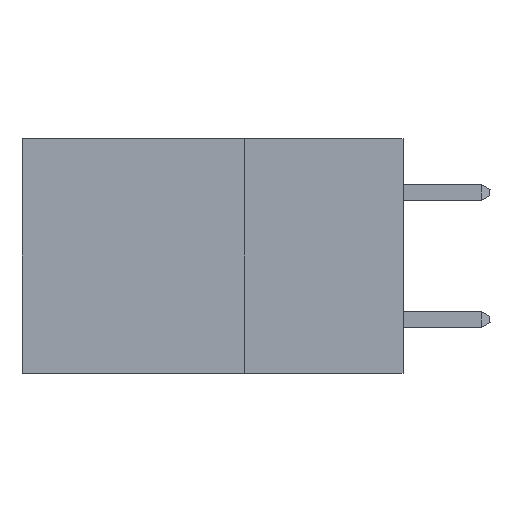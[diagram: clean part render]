
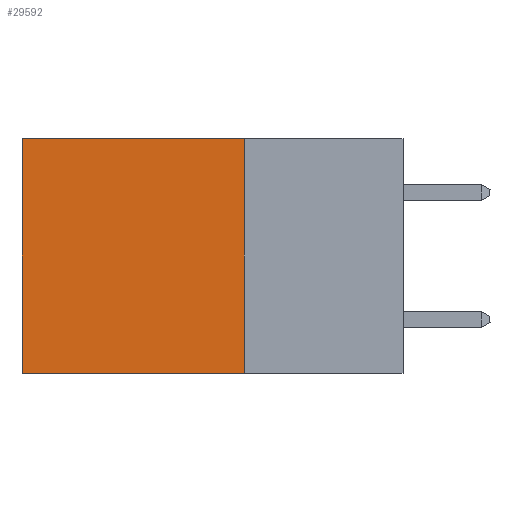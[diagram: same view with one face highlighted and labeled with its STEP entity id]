
A CAD part, left-side view. The second image highlights one B-rep face of the part: STEP entity #29592.
In plain terms, the highlighted planar face has unit normal (-1, 0, 0).
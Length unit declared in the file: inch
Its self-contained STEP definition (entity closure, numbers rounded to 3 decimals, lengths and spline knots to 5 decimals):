
#1355 = ORIENTED_EDGE ( 'NONE', *, *, #19962, .T. ) ;
#1936 = FACE_OUTER_BOUND ( 'NONE', #5092, .T. ) ;
#2747 = VECTOR ( 'NONE', #10134, 39.37008 ) ;
#3087 = DIRECTION ( 'NONE',  ( 0., 1., 0. ) ) ;
#3748 = VECTOR ( 'NONE', #14158, 39.37008 ) ;
#5092 = EDGE_LOOP ( 'NONE', ( #1355, #26236, #13991, #19894 ) ) ;
#6205 = VERTEX_POINT ( 'NONE', #20364 ) ;
#6422 = EDGE_CURVE ( 'NONE', #6205, #20062, #10120, .T. ) ;
#7915 = CARTESIAN_POINT ( 'NONE',  ( 0.2875, 0.25, 0. ) ) ;
#8885 = LINE ( 'NONE', #30824, #30313 ) ;
#9752 = VERTEX_POINT ( 'NONE', #24562 ) ;
#10120 = LINE ( 'NONE', #21215, #2747 ) ;
#10134 = DIRECTION ( 'NONE',  ( 0., 1., 0. ) ) ;
#10669 = DIRECTION ( 'NONE',  ( 0., 0., -1. ) ) ;
#13991 = ORIENTED_EDGE ( 'NONE', *, *, #21812, .F. ) ;
#14158 = DIRECTION ( 'NONE',  ( 0., 0., -1. ) ) ;
#16784 = DIRECTION ( 'NONE',  ( 0., 0., -1. ) ) ;
#17314 = CARTESIAN_POINT ( 'NONE',  ( 0.2875, 0.6, -0.37 ) ) ;
#17610 = LINE ( 'NONE', #22634, #3748 ) ;
#19894 = ORIENTED_EDGE ( 'NONE', *, *, #30751, .T. ) ;
#19962 = EDGE_CURVE ( 'NONE', #21823, #20062, #17610, .T. ) ;
#20062 = VERTEX_POINT ( 'NONE', #17314 ) ;
#20364 = CARTESIAN_POINT ( 'NONE',  ( 0.2875, 0.25, -0.37 ) ) ;
#21215 = CARTESIAN_POINT ( 'NONE',  ( 0.2875, 0.25, -0.37 ) ) ;
#21812 = EDGE_CURVE ( 'NONE', #9752, #6205, #8885, .T. ) ;
#21823 = VERTEX_POINT ( 'NONE', #25307 ) ;
#22634 = CARTESIAN_POINT ( 'NONE',  ( 0.2875, 0.6, 0. ) ) ;
#24562 = CARTESIAN_POINT ( 'NONE',  ( 0.2875, 0.25, 0. ) ) ;
#25307 = CARTESIAN_POINT ( 'NONE',  ( 0.2875, 0.6, 0. ) ) ;
#26236 = ORIENTED_EDGE ( 'NONE', *, *, #6422, .F. ) ;
#27453 = DIRECTION ( 'NONE',  ( 1., 0., 0. ) ) ;
#27942 = AXIS2_PLACEMENT_3D ( 'NONE', #7915, #27453, #10669 ) ;
#28247 = CARTESIAN_POINT ( 'NONE',  ( 0.2875, 0.25, 0. ) ) ;
#29592 = ADVANCED_FACE ( 'NONE', ( #1936 ), #30155, .F. ) ;
#29708 = LINE ( 'NONE', #28247, #35275 ) ;
#30155 = PLANE ( 'NONE',  #27942 ) ;
#30313 = VECTOR ( 'NONE', #16784, 39.37008 ) ;
#30751 = EDGE_CURVE ( 'NONE', #9752, #21823, #29708, .T. ) ;
#30824 = CARTESIAN_POINT ( 'NONE',  ( 0.2875, 0.25, 0. ) ) ;
#35275 = VECTOR ( 'NONE', #3087, 39.37008 ) ;
